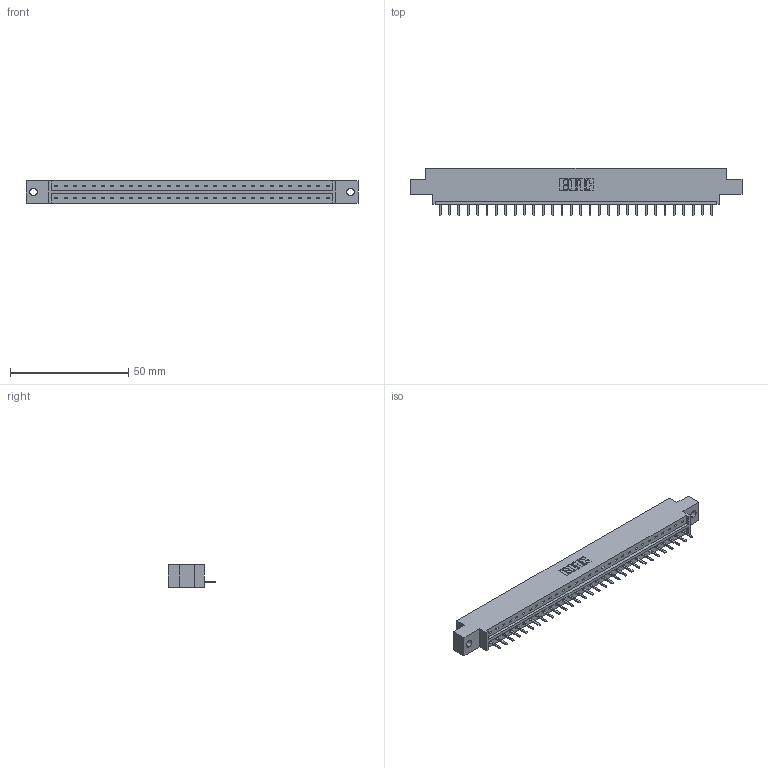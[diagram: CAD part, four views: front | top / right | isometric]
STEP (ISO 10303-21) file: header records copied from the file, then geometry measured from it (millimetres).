
FILE_DESCRIPTION (( 'STEP AP203' ), '1' );
FILE_NAME ('333-030-520-602.STEP', '2018-08-02T17:11:18', ( '' ), ( '' ), 'SwSTEP 2.0', 'SolidWorks 2016', '' );
FILE_SCHEMA (( 'CONFIG_CONTROL_DESIGN' ));
Length unit declared in the file: inch
Products named in the file (3): 345-292-001_345-293-120; 333-030-520-602; 333 Part_Offset - .128 Dia
Assembly tree (31 placements, depth 2):
  333-030-520-602
    333 Part_Offset - .128 Dia
    345-292-001_345-293-120  x30
Bounding box: 140.41 x 20.02 x 9.4 mm (x, y, z)
Volume: 13675.4 mm3; surface area: 14341 mm2
Topology: 31 solids, 31 shells, 1978 faces, 5843 edges, 3814 vertices
Faces by surface type: plane 1394, cylinder 584
Entity records: 20141 total; most frequent: CARTESIAN_POINT 3496, ORIENTED_EDGE 3450, DIRECTION 2961, EDGE_CURVE 1725, VECTOR 1593, LINE 1593, VERTEX_POINT 1146, AXIS2_PLACEMENT_3D 684
